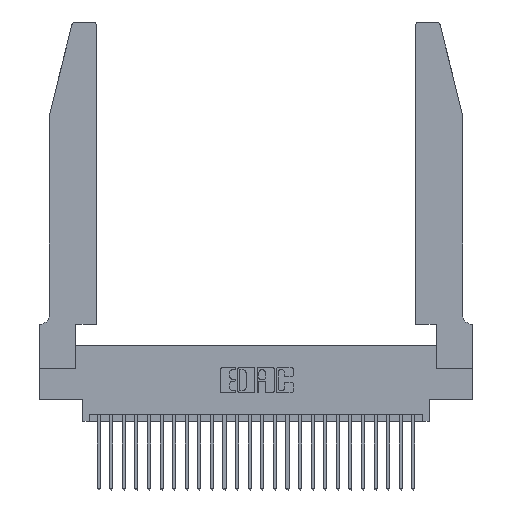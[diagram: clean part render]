
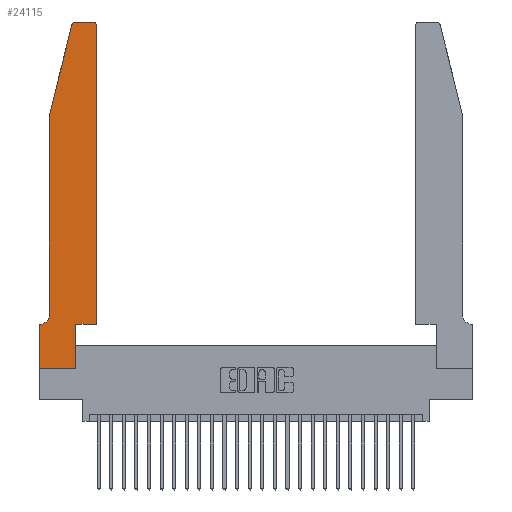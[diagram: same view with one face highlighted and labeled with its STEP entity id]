
A CAD part, top view. The second image highlights one B-rep face of the part: STEP entity #24115.
In plain terms, the highlighted planar face has unit normal (0, 0, 1).
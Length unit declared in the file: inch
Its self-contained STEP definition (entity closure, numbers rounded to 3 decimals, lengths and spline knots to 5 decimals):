
#233 = AXIS2_PLACEMENT_3D ( 'NONE', #2614, #15474, #9061 ) ;
#613 = EDGE_CURVE ( 'NONE', #9559, #901, #24412, .T. ) ;
#627 = EDGE_CURVE ( 'NONE', #15303, #8963, #13132, .T. ) ;
#901 = VERTEX_POINT ( 'NONE', #18096 ) ;
#1165 = DIRECTION ( 'NONE',  ( -1., 0., 0. ) ) ;
#1304 = VERTEX_POINT ( 'NONE', #25737 ) ;
#1329 = ORIENTED_EDGE ( 'NONE', *, *, #23714, .T. ) ;
#1379 = VERTEX_POINT ( 'NONE', #10949 ) ;
#1405 = DIRECTION ( 'NONE',  ( 0., 1., 0. ) ) ;
#1623 = LINE ( 'NONE', #7978, #20556 ) ;
#1658 = EDGE_CURVE ( 'NONE', #23102, #17743, #10467, .T. ) ;
#1970 = CIRCLE ( 'NONE', #3017, 0.03 ) ;
#2104 = CARTESIAN_POINT ( 'NONE',  ( 0.284, 2.72, 0.37 ) ) ;
#2163 = VERTEX_POINT ( 'NONE', #5807 ) ;
#2385 = CARTESIAN_POINT ( 'NONE',  ( 0.0755, 2., 0.37 ) ) ;
#2614 = CARTESIAN_POINT ( 'NONE',  ( 0.4205, 2.72, 0.37 ) ) ;
#2908 = AXIS2_PLACEMENT_3D ( 'NONE', #3509, #12143, #24723 ) ;
#2954 = EDGE_CURVE ( 'NONE', #901, #23102, #10393, .T. ) ;
#3017 = AXIS2_PLACEMENT_3D ( 'NONE', #2104, #12510, #10316 ) ;
#3031 = LINE ( 'NONE', #27324, #17249 ) ;
#3450 = ORIENTED_EDGE ( 'NONE', *, *, #11376, .T. ) ;
#3509 = CARTESIAN_POINT ( 'NONE',  ( 0.0055, 0.42, 0.37 ) ) ;
#3627 = CARTESIAN_POINT ( 'NONE',  ( 0.25487, 2.72718, 0.37 ) ) ;
#5408 = CARTESIAN_POINT ( 'NONE',  ( 0.2865, 0.35, 0.37 ) ) ;
#5451 = ORIENTED_EDGE ( 'NONE', *, *, #613, .T. ) ;
#5604 = ORIENTED_EDGE ( 'NONE', *, *, #1658, .T. ) ;
#5807 = CARTESIAN_POINT ( 'NONE',  ( 0.284, 2.75, 0.37 ) ) ;
#6214 = LINE ( 'NONE', #9094, #22448 ) ;
#6704 = DIRECTION ( 'NONE',  ( -0.239, -0.971, 0. ) ) ;
#7124 = EDGE_CURVE ( 'NONE', #23222, #9116, #3031, .T. ) ;
#7821 = DIRECTION ( 'NONE',  ( 0., -1., 0. ) ) ;
#7901 = CARTESIAN_POINT ( 'NONE',  ( 0.0755, 0.42, 0.37 ) ) ;
#7978 = CARTESIAN_POINT ( 'NONE',  ( 0.2865, 0.35, 0.37 ) ) ;
#8530 = ORIENTED_EDGE ( 'NONE', *, *, #25261, .T. ) ;
#8881 = VECTOR ( 'NONE', #1165, 39.37008 ) ;
#8963 = VERTEX_POINT ( 'NONE', #14714 ) ;
#9060 = CARTESIAN_POINT ( 'NONE',  ( 0., 0., 0.37 ) ) ;
#9061 = DIRECTION ( 'NONE',  ( 1., 0., 0. ) ) ;
#9094 = CARTESIAN_POINT ( 'NONE',  ( 0.2605, 2.75, 0.37 ) ) ;
#9116 = VERTEX_POINT ( 'NONE', #10177 ) ;
#9427 = ORIENTED_EDGE ( 'NONE', *, *, #23836, .T. ) ;
#9541 = LINE ( 'NONE', #26108, #8881 ) ;
#9559 = VERTEX_POINT ( 'NONE', #5408 ) ;
#9748 = DIRECTION ( 'NONE',  ( 0., 1., 0. ) ) ;
#10177 = CARTESIAN_POINT ( 'NONE',  ( 0., 0., 0.37 ) ) ;
#10188 = AXIS2_PLACEMENT_3D ( 'NONE', #24441, #18057, #13585 ) ;
#10316 = DIRECTION ( 'NONE',  ( 1., 0., 0. ) ) ;
#10393 = LINE ( 'NONE', #24687, #11695 ) ;
#10467 = CIRCLE ( 'NONE', #233, 0.03 ) ;
#10719 = CARTESIAN_POINT ( 'NONE',  ( 0.0755, 2., 0.37 ) ) ;
#10949 = CARTESIAN_POINT ( 'NONE',  ( 0.2865, 0., 0.37 ) ) ;
#11320 = CIRCLE ( 'NONE', #2908, 0.07 ) ;
#11376 = EDGE_CURVE ( 'NONE', #15219, #1304, #11320, .T. ) ;
#11695 = VECTOR ( 'NONE', #1405, 39.37008 ) ;
#12064 = ORIENTED_EDGE ( 'NONE', *, *, #15968, .T. ) ;
#12143 = DIRECTION ( 'NONE',  ( 0., 0., -1. ) ) ;
#12510 = DIRECTION ( 'NONE',  ( 0., 0., 1. ) ) ;
#12549 = CARTESIAN_POINT ( 'NONE',  ( 0.4505, 2.72, 0.37 ) ) ;
#12782 = DIRECTION ( 'NONE',  ( 0., -1., 0. ) ) ;
#13057 = VECTOR ( 'NONE', #12782, 39.37008 ) ;
#13132 = LINE ( 'NONE', #10719, #20111 ) ;
#13173 = DIRECTION ( 'NONE',  ( 1., 0., 0. ) ) ;
#13463 = DIRECTION ( 'NONE',  ( 1., 0., 0. ) ) ;
#13585 = DIRECTION ( 'NONE',  ( 1., 0., 0. ) ) ;
#13953 = EDGE_CURVE ( 'NONE', #17743, #2163, #6214, .T. ) ;
#14714 = CARTESIAN_POINT ( 'NONE',  ( 0.0755, 2., 0.37 ) ) ;
#15219 = VERTEX_POINT ( 'NONE', #7901 ) ;
#15303 = VERTEX_POINT ( 'NONE', #3627 ) ;
#15474 = DIRECTION ( 'NONE',  ( 0., 0., 1. ) ) ;
#15483 = EDGE_CURVE ( 'NONE', #8963, #15219, #25970, .T. ) ;
#15847 = ORIENTED_EDGE ( 'NONE', *, *, #627, .T. ) ;
#15968 = EDGE_CURVE ( 'NONE', #9116, #1379, #17011, .T. ) ;
#17011 = LINE ( 'NONE', #9060, #18688 ) ;
#17249 = VECTOR ( 'NONE', #7821, 39.37008 ) ;
#17743 = VERTEX_POINT ( 'NONE', #23659 ) ;
#18057 = DIRECTION ( 'NONE',  ( 0., 0., 1. ) ) ;
#18096 = CARTESIAN_POINT ( 'NONE',  ( 0.4505, 0.35, 0.37 ) ) ;
#18620 = ORIENTED_EDGE ( 'NONE', *, *, #2954, .T. ) ;
#18688 = VECTOR ( 'NONE', #13463, 39.37008 ) ;
#19832 = EDGE_LOOP ( 'NONE', ( #23492, #9427, #15847, #22762, #3450, #8530, #22412, #12064, #1329, #5451, #18620, #5604 ) ) ;
#20094 = PLANE ( 'NONE',  #10188 ) ;
#20111 = VECTOR ( 'NONE', #6704, 39.37008 ) ;
#20556 = VECTOR ( 'NONE', #9748, 39.37008 ) ;
#21434 = VECTOR ( 'NONE', #13173, 39.37008 ) ;
#22412 = ORIENTED_EDGE ( 'NONE', *, *, #7124, .T. ) ;
#22448 = VECTOR ( 'NONE', #23883, 39.37008 ) ;
#22762 = ORIENTED_EDGE ( 'NONE', *, *, #15483, .T. ) ;
#23102 = VERTEX_POINT ( 'NONE', #12549 ) ;
#23222 = VERTEX_POINT ( 'NONE', #24954 ) ;
#23367 = CARTESIAN_POINT ( 'NONE',  ( 0.4505, 0.35, 0.37 ) ) ;
#23492 = ORIENTED_EDGE ( 'NONE', *, *, #13953, .T. ) ;
#23659 = CARTESIAN_POINT ( 'NONE',  ( 0.4205, 2.75, 0.37 ) ) ;
#23714 = EDGE_CURVE ( 'NONE', #1379, #9559, #1623, .T. ) ;
#23828 = FACE_OUTER_BOUND ( 'NONE', #19832, .T. ) ;
#23836 = EDGE_CURVE ( 'NONE', #2163, #15303, #1970, .T. ) ;
#23883 = DIRECTION ( 'NONE',  ( -1., 0., 0. ) ) ;
#24115 = ADVANCED_FACE ( 'NONE', ( #23828 ), #20094, .T. ) ;
#24412 = LINE ( 'NONE', #23367, #21434 ) ;
#24441 = CARTESIAN_POINT ( 'NONE',  ( 0., 0.35, 0.37 ) ) ;
#24687 = CARTESIAN_POINT ( 'NONE',  ( 0.4505, 0.35, 0.37 ) ) ;
#24723 = DIRECTION ( 'NONE',  ( -1., 0., 0. ) ) ;
#24954 = CARTESIAN_POINT ( 'NONE',  ( 0., 0.35, 0.37 ) ) ;
#25261 = EDGE_CURVE ( 'NONE', #1304, #23222, #9541, .T. ) ;
#25737 = CARTESIAN_POINT ( 'NONE',  ( 0.0055, 0.35, 0.37 ) ) ;
#25970 = LINE ( 'NONE', #2385, #13057 ) ;
#26108 = CARTESIAN_POINT ( 'NONE',  ( 0.0755, 0.35, 0.37 ) ) ;
#27324 = CARTESIAN_POINT ( 'NONE',  ( 0., 0., 0.37 ) ) ;
